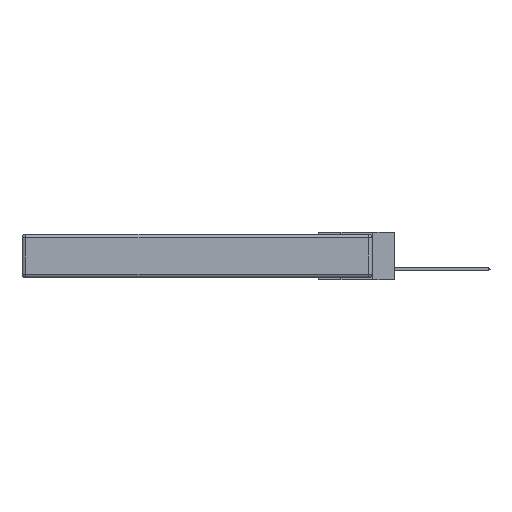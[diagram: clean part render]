
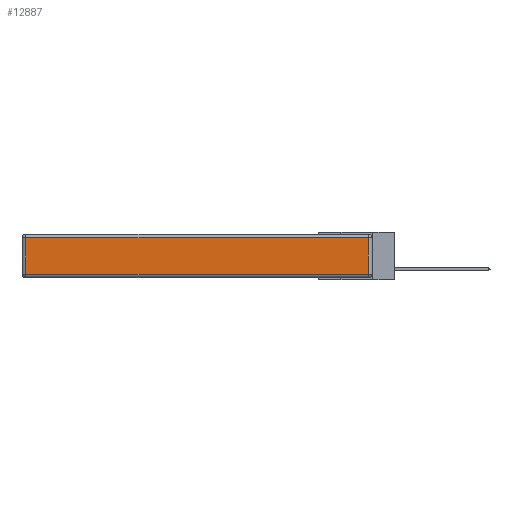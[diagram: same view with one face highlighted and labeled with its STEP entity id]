
A CAD part, left-side view. The second image highlights one B-rep face of the part: STEP entity #12887.
In plain terms, the highlighted planar face has unit normal (-1, 0, 0).
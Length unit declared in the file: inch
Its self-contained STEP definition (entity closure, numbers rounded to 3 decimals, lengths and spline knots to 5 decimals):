
#71 = VERTEX_POINT ( 'NONE', #12852 ) ;
#270 = DIRECTION ( 'NONE',  ( 0., 1., 0. ) ) ;
#1179 = VERTEX_POINT ( 'NONE', #5102 ) ;
#1664 = CARTESIAN_POINT ( 'NONE',  ( 0., 2.75, -0.03 ) ) ;
#3116 = ORIENTED_EDGE ( 'NONE', *, *, #5756, .T. ) ;
#3662 = VECTOR ( 'NONE', #270, 39.37008 ) ;
#3692 = CARTESIAN_POINT ( 'NONE',  ( 0., 0.03, -0.03 ) ) ;
#3931 = DIRECTION ( 'NONE',  ( 0., 0., 1. ) ) ;
#4185 = PLANE ( 'NONE',  #11363 ) ;
#4513 = DIRECTION ( 'NONE',  ( 0., -1., 0. ) ) ;
#4660 = FACE_OUTER_BOUND ( 'NONE', #7987, .T. ) ;
#4676 = LINE ( 'NONE', #1664, #3662 ) ;
#4741 = EDGE_CURVE ( 'NONE', #1179, #15394, #6684, .T. ) ;
#5102 = CARTESIAN_POINT ( 'NONE',  ( 0., 2.72, -0.03 ) ) ;
#5455 = CARTESIAN_POINT ( 'NONE',  ( 0., 0., -0.343 ) ) ;
#5572 = DIRECTION ( 'NONE',  ( 0., 0., 1. ) ) ;
#5756 = EDGE_CURVE ( 'NONE', #15394, #71, #8863, .T. ) ;
#6209 = CARTESIAN_POINT ( 'NONE',  ( 0., 2.72, -0.313 ) ) ;
#6684 = LINE ( 'NONE', #10141, #10516 ) ;
#6750 = ORIENTED_EDGE ( 'NONE', *, *, #4741, .T. ) ;
#7987 = EDGE_LOOP ( 'NONE', ( #3116, #8197, #15385, #6750 ) ) ;
#8197 = ORIENTED_EDGE ( 'NONE', *, *, #11254, .T. ) ;
#8863 = LINE ( 'NONE', #13297, #10082 ) ;
#10061 = EDGE_CURVE ( 'NONE', #10177, #1179, #4676, .T. ) ;
#10082 = VECTOR ( 'NONE', #4513, 39.37008 ) ;
#10141 = CARTESIAN_POINT ( 'NONE',  ( 0., 2.72, -0.343 ) ) ;
#10177 = VERTEX_POINT ( 'NONE', #3692 ) ;
#10516 = VECTOR ( 'NONE', #13990, 39.37008 ) ;
#10533 = DIRECTION ( 'NONE',  ( -1., 0., 0. ) ) ;
#10548 = VECTOR ( 'NONE', #3931, 39.37008 ) ;
#11254 = EDGE_CURVE ( 'NONE', #71, #10177, #13941, .T. ) ;
#11363 = AXIS2_PLACEMENT_3D ( 'NONE', #5455, #10533, #5572 ) ;
#12852 = CARTESIAN_POINT ( 'NONE',  ( 0., 0.03, -0.313 ) ) ;
#12887 = ADVANCED_FACE ( 'NONE', ( #4660 ), #4185, .T. ) ;
#13297 = CARTESIAN_POINT ( 'NONE',  ( 0., 0., -0.313 ) ) ;
#13941 = LINE ( 'NONE', #14081, #10548 ) ;
#13990 = DIRECTION ( 'NONE',  ( 0., 0., -1. ) ) ;
#14081 = CARTESIAN_POINT ( 'NONE',  ( 0., 0.03, -0.343 ) ) ;
#15385 = ORIENTED_EDGE ( 'NONE', *, *, #10061, .T. ) ;
#15394 = VERTEX_POINT ( 'NONE', #6209 ) ;
